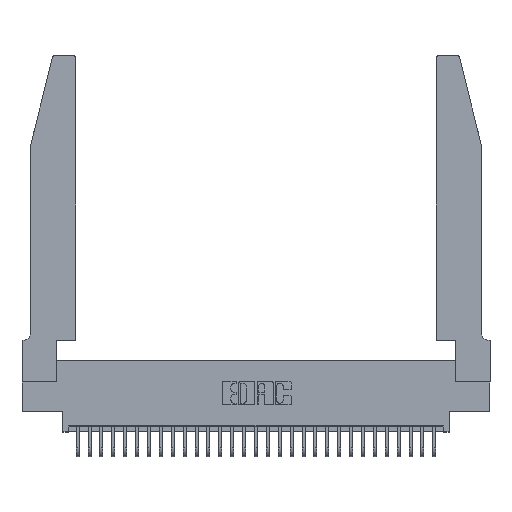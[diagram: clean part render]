
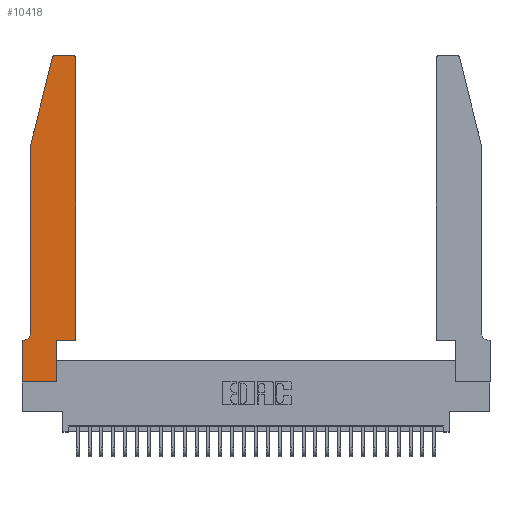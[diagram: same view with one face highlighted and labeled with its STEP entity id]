
A CAD part, top view. The second image highlights one B-rep face of the part: STEP entity #10418.
In plain terms, the highlighted planar face has unit normal (0, 0, 1).
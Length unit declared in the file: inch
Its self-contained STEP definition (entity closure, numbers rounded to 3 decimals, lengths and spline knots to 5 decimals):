
#179 = CARTESIAN_POINT ( 'NONE',  ( 0.284, 2.75, 0.37 ) ) ;
#1214 = FACE_OUTER_BOUND ( 'NONE', #32005, .T. ) ;
#1266 = VERTEX_POINT ( 'NONE', #9219 ) ;
#1648 = CARTESIAN_POINT ( 'NONE',  ( 0.2865, 0.35, 0.37 ) ) ;
#1659 = VERTEX_POINT ( 'NONE', #30553 ) ;
#1697 = DIRECTION ( 'NONE',  ( 1., 0., 0. ) ) ;
#1729 = ORIENTED_EDGE ( 'NONE', *, *, #8416, .T. ) ;
#2209 = CARTESIAN_POINT ( 'NONE',  ( 0.0755, 0.42, 0.37 ) ) ;
#2243 = DIRECTION ( 'NONE',  ( 0., 1., 0. ) ) ;
#2250 = CARTESIAN_POINT ( 'NONE',  ( 0., 0., 0.37 ) ) ;
#3845 = DIRECTION ( 'NONE',  ( 0., 0., 1. ) ) ;
#3961 = VECTOR ( 'NONE', #17226, 39.37008 ) ;
#5162 = ORIENTED_EDGE ( 'NONE', *, *, #10333, .T. ) ;
#6048 = VECTOR ( 'NONE', #2243, 39.37008 ) ;
#6060 = DIRECTION ( 'NONE',  ( 1., 0., 0. ) ) ;
#6162 = CARTESIAN_POINT ( 'NONE',  ( 0.284, 2.72, 0.37 ) ) ;
#6511 = CARTESIAN_POINT ( 'NONE',  ( 0., 0., 0.37 ) ) ;
#6579 = CARTESIAN_POINT ( 'NONE',  ( 0.0755, 0.35, 0.37 ) ) ;
#7260 = VERTEX_POINT ( 'NONE', #179 ) ;
#7325 = VERTEX_POINT ( 'NONE', #7845 ) ;
#7409 = DIRECTION ( 'NONE',  ( 1., 0., 0. ) ) ;
#7618 = CARTESIAN_POINT ( 'NONE',  ( 0.4505, 2.72, 0.37 ) ) ;
#7845 = CARTESIAN_POINT ( 'NONE',  ( 0.2865, 0.35, 0.37 ) ) ;
#8169 = EDGE_CURVE ( 'NONE', #9746, #31865, #31859, .T. ) ;
#8416 = EDGE_CURVE ( 'NONE', #27496, #7260, #29890, .T. ) ;
#8593 = CARTESIAN_POINT ( 'NONE',  ( 0.0755, 2., 0.37 ) ) ;
#8913 = DIRECTION ( 'NONE',  ( 0., 0., 1. ) ) ;
#9052 = LINE ( 'NONE', #2250, #15674 ) ;
#9219 = CARTESIAN_POINT ( 'NONE',  ( 0.0055, 0.35, 0.37 ) ) ;
#9377 = EDGE_CURVE ( 'NONE', #12276, #7325, #25154, .T. ) ;
#9450 = CARTESIAN_POINT ( 'NONE',  ( 0.4205, 2.72, 0.37 ) ) ;
#9504 = CARTESIAN_POINT ( 'NONE',  ( 0.0755, 2., 0.37 ) ) ;
#9746 = VERTEX_POINT ( 'NONE', #13769 ) ;
#10146 = ORIENTED_EDGE ( 'NONE', *, *, #27422, .T. ) ;
#10333 = EDGE_CURVE ( 'NONE', #27888, #9746, #23114, .T. ) ;
#10418 = ADVANCED_FACE ( 'NONE', ( #1214 ), #31629, .T. ) ;
#11812 = DIRECTION ( 'NONE',  ( 1., 0., 0. ) ) ;
#11983 = DIRECTION ( 'NONE',  ( 1., 0., 0. ) ) ;
#12168 = AXIS2_PLACEMENT_3D ( 'NONE', #6162, #3845, #6060 ) ;
#12256 = EDGE_CURVE ( 'NONE', #7325, #30262, #25365, .T. ) ;
#12276 = VERTEX_POINT ( 'NONE', #16485 ) ;
#13769 = CARTESIAN_POINT ( 'NONE',  ( 0.0755, 2., 0.37 ) ) ;
#14344 = DIRECTION ( 'NONE',  ( 0., 1., 0. ) ) ;
#14862 = ORIENTED_EDGE ( 'NONE', *, *, #9377, .T. ) ;
#15377 = ORIENTED_EDGE ( 'NONE', *, *, #12256, .T. ) ;
#15674 = VECTOR ( 'NONE', #7409, 39.37008 ) ;
#15709 = DIRECTION ( 'NONE',  ( -1., 0., 0. ) ) ;
#15874 = CARTESIAN_POINT ( 'NONE',  ( 0.4505, 0.35, 0.37 ) ) ;
#15953 = EDGE_CURVE ( 'NONE', #31865, #1266, #26761, .T. ) ;
#16080 = DIRECTION ( 'NONE',  ( -1., 0., 0. ) ) ;
#16122 = ORIENTED_EDGE ( 'NONE', *, *, #26808, .T. ) ;
#16485 = CARTESIAN_POINT ( 'NONE',  ( 0.2865, 0., 0.37 ) ) ;
#16541 = VERTEX_POINT ( 'NONE', #7618 ) ;
#16631 = DIRECTION ( 'NONE',  ( 0., 0., -1. ) ) ;
#16687 = VERTEX_POINT ( 'NONE', #6511 ) ;
#17158 = CIRCLE ( 'NONE', #12168, 0.03 ) ;
#17226 = DIRECTION ( 'NONE',  ( 0., -1., 0. ) ) ;
#18026 = EDGE_CURVE ( 'NONE', #1659, #16687, #23525, .T. ) ;
#18342 = CIRCLE ( 'NONE', #31797, 0.03 ) ;
#18508 = VECTOR ( 'NONE', #14344, 39.37008 ) ;
#18640 = DIRECTION ( 'NONE',  ( -0.239, -0.971, 0. ) ) ;
#19096 = CARTESIAN_POINT ( 'NONE',  ( 0.4505, 0.35, 0.37 ) ) ;
#19108 = ORIENTED_EDGE ( 'NONE', *, *, #32235, .T. ) ;
#19335 = VECTOR ( 'NONE', #22135, 39.37008 ) ;
#19453 = EDGE_CURVE ( 'NONE', #7260, #27888, #17158, .T. ) ;
#19495 = VECTOR ( 'NONE', #11812, 39.37008 ) ;
#20054 = ORIENTED_EDGE ( 'NONE', *, *, #24432, .T. ) ;
#20207 = CARTESIAN_POINT ( 'NONE',  ( 0.4205, 2.75, 0.37 ) ) ;
#21157 = AXIS2_PLACEMENT_3D ( 'NONE', #28998, #8913, #1697 ) ;
#21527 = CARTESIAN_POINT ( 'NONE',  ( 0.0055, 0.42, 0.37 ) ) ;
#22135 = DIRECTION ( 'NONE',  ( 0., -1., 0. ) ) ;
#22982 = VECTOR ( 'NONE', #16080, 39.37008 ) ;
#23114 = LINE ( 'NONE', #8593, #28579 ) ;
#23525 = LINE ( 'NONE', #32286, #3961 ) ;
#23579 = ORIENTED_EDGE ( 'NONE', *, *, #8169, .T. ) ;
#23935 = CARTESIAN_POINT ( 'NONE',  ( 0.25487, 2.72718, 0.37 ) ) ;
#24372 = ORIENTED_EDGE ( 'NONE', *, *, #18026, .T. ) ;
#24432 = EDGE_CURVE ( 'NONE', #30262, #16541, #25961, .T. ) ;
#24572 = LINE ( 'NONE', #6579, #22982 ) ;
#24768 = CARTESIAN_POINT ( 'NONE',  ( 0.4505, 0.35, 0.37 ) ) ;
#25154 = LINE ( 'NONE', #1648, #18508 ) ;
#25365 = LINE ( 'NONE', #19096, #19495 ) ;
#25961 = LINE ( 'NONE', #24768, #6048 ) ;
#26761 = CIRCLE ( 'NONE', #29631, 0.07 ) ;
#26808 = EDGE_CURVE ( 'NONE', #16687, #12276, #9052, .T. ) ;
#26903 = DIRECTION ( 'NONE',  ( 0., 0., 1. ) ) ;
#27422 = EDGE_CURVE ( 'NONE', #16541, #27496, #18342, .T. ) ;
#27496 = VERTEX_POINT ( 'NONE', #20207 ) ;
#27888 = VERTEX_POINT ( 'NONE', #23935 ) ;
#28579 = VECTOR ( 'NONE', #18640, 39.37008 ) ;
#28998 = CARTESIAN_POINT ( 'NONE',  ( 0., 0.35, 0.37 ) ) ;
#29282 = DIRECTION ( 'NONE',  ( -1., 0., 0. ) ) ;
#29294 = ORIENTED_EDGE ( 'NONE', *, *, #19453, .T. ) ;
#29631 = AXIS2_PLACEMENT_3D ( 'NONE', #21527, #16631, #29282 ) ;
#29890 = LINE ( 'NONE', #30869, #31826 ) ;
#30262 = VERTEX_POINT ( 'NONE', #15874 ) ;
#30553 = CARTESIAN_POINT ( 'NONE',  ( 0., 0.35, 0.37 ) ) ;
#30869 = CARTESIAN_POINT ( 'NONE',  ( 0.2605, 2.75, 0.37 ) ) ;
#31507 = ORIENTED_EDGE ( 'NONE', *, *, #15953, .T. ) ;
#31629 = PLANE ( 'NONE',  #21157 ) ;
#31797 = AXIS2_PLACEMENT_3D ( 'NONE', #9450, #26903, #11983 ) ;
#31826 = VECTOR ( 'NONE', #15709, 39.37008 ) ;
#31859 = LINE ( 'NONE', #9504, #19335 ) ;
#31865 = VERTEX_POINT ( 'NONE', #2209 ) ;
#32005 = EDGE_LOOP ( 'NONE', ( #1729, #29294, #5162, #23579, #31507, #19108, #24372, #16122, #14862, #15377, #20054, #10146 ) ) ;
#32235 = EDGE_CURVE ( 'NONE', #1266, #1659, #24572, .T. ) ;
#32286 = CARTESIAN_POINT ( 'NONE',  ( 0., 0., 0.37 ) ) ;
